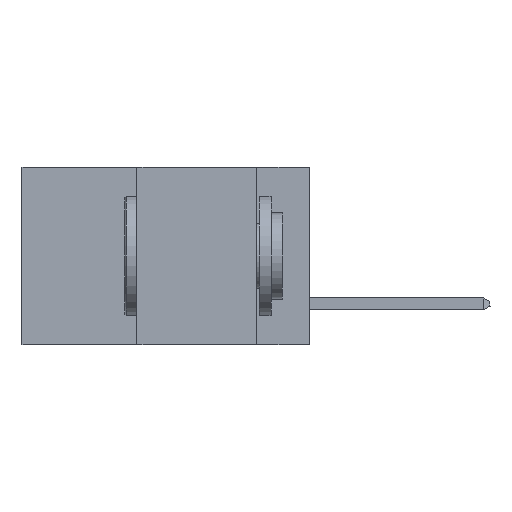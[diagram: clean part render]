
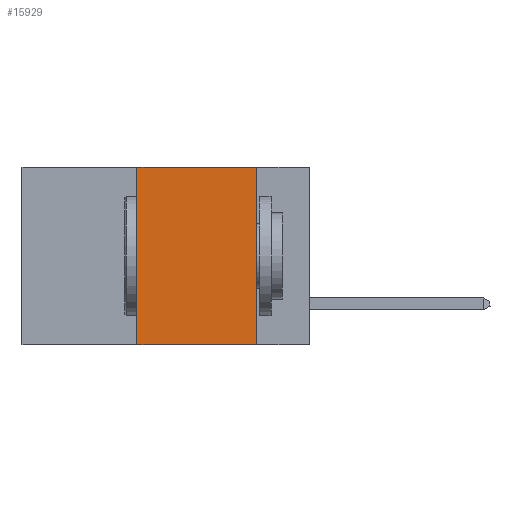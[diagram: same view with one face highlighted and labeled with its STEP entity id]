
A CAD part, left-side view. The second image highlights one B-rep face of the part: STEP entity #15929.
In plain terms, the highlighted planar face has unit normal (-1, 0, 0).
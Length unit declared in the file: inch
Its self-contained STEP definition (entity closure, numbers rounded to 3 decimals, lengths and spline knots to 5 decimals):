
#276 = VERTEX_POINT ( 'NONE', #2988 ) ;
#1346 = VERTEX_POINT ( 'NONE', #8165 ) ;
#1421 = VERTEX_POINT ( 'NONE', #5928 ) ;
#2020 = CARTESIAN_POINT ( 'NONE',  ( 0., 0.36, 0. ) ) ;
#2033 = VECTOR ( 'NONE', #5531, 39.37008 ) ;
#2090 = DIRECTION ( 'NONE',  ( 0., 0., 1. ) ) ;
#2442 = PLANE ( 'NONE',  #10254 ) ;
#2493 = FACE_OUTER_BOUND ( 'NONE', #3020, .T. ) ;
#2988 = CARTESIAN_POINT ( 'NONE',  ( 0., 0.11, 0. ) ) ;
#3020 = EDGE_LOOP ( 'NONE', ( #6273, #8714, #5689, #3616 ) ) ;
#3616 = ORIENTED_EDGE ( 'NONE', *, *, #5652, .T. ) ;
#3868 = DIRECTION ( 'NONE',  ( 0., 0., -1. ) ) ;
#5531 = DIRECTION ( 'NONE',  ( 0., 0., -1. ) ) ;
#5542 = DIRECTION ( 'NONE',  ( 1., 0., 0. ) ) ;
#5652 = EDGE_CURVE ( 'NONE', #12061, #1346, #14513, .T. ) ;
#5689 = ORIENTED_EDGE ( 'NONE', *, *, #15022, .F. ) ;
#5928 = CARTESIAN_POINT ( 'NONE',  ( 0., 0.36, 0. ) ) ;
#6273 = ORIENTED_EDGE ( 'NONE', *, *, #7932, .F. ) ;
#6516 = LINE ( 'NONE', #10202, #2033 ) ;
#7932 = EDGE_CURVE ( 'NONE', #276, #1346, #6516, .T. ) ;
#8165 = CARTESIAN_POINT ( 'NONE',  ( 0., 0.11, -0.37 ) ) ;
#8297 = CARTESIAN_POINT ( 'NONE',  ( 0., 0.6, -0.37 ) ) ;
#8714 = ORIENTED_EDGE ( 'NONE', *, *, #9640, .F. ) ;
#8944 = DIRECTION ( 'NONE',  ( 0., -1., 0. ) ) ;
#9640 = EDGE_CURVE ( 'NONE', #1421, #276, #19153, .T. ) ;
#10202 = CARTESIAN_POINT ( 'NONE',  ( 0., 0.11, 0. ) ) ;
#10254 = AXIS2_PLACEMENT_3D ( 'NONE', #19808, #5542, #3868 ) ;
#12061 = VERTEX_POINT ( 'NONE', #16306 ) ;
#13952 = LINE ( 'NONE', #2020, #19183 ) ;
#14436 = DIRECTION ( 'NONE',  ( 0., -1., 0. ) ) ;
#14513 = LINE ( 'NONE', #8297, #19484 ) ;
#14859 = CARTESIAN_POINT ( 'NONE',  ( 0., 0.6, 0. ) ) ;
#15022 = EDGE_CURVE ( 'NONE', #12061, #1421, #13952, .T. ) ;
#15651 = VECTOR ( 'NONE', #8944, 39.37008 ) ;
#15929 = ADVANCED_FACE ( 'NONE', ( #2493 ), #2442, .F. ) ;
#16306 = CARTESIAN_POINT ( 'NONE',  ( 0., 0.36, -0.37 ) ) ;
#19153 = LINE ( 'NONE', #14859, #15651 ) ;
#19183 = VECTOR ( 'NONE', #2090, 39.37008 ) ;
#19484 = VECTOR ( 'NONE', #14436, 39.37008 ) ;
#19808 = CARTESIAN_POINT ( 'NONE',  ( 0., 0.6, 0. ) ) ;
